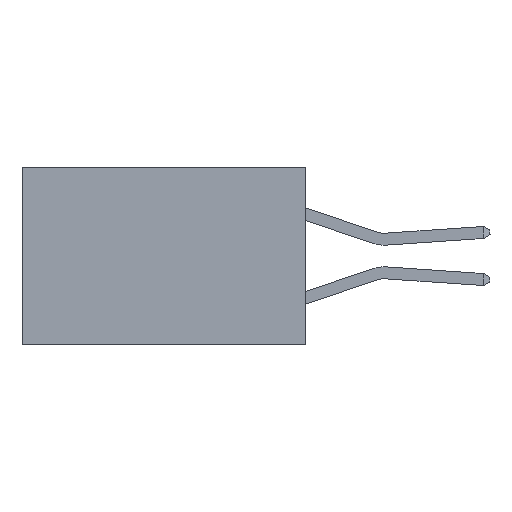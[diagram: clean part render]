
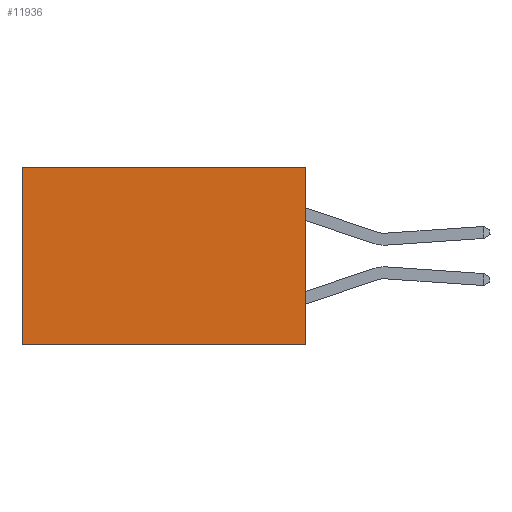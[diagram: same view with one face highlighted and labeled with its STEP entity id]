
A CAD part, left-side view. The second image highlights one B-rep face of the part: STEP entity #11936.
In plain terms, the highlighted planar face has unit normal (-1, 0, 0).
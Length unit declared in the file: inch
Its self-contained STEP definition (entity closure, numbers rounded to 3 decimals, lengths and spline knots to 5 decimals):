
#502 = ORIENTED_EDGE ( 'NONE', *, *, #6979, .T. ) ;
#2193 = AXIS2_PLACEMENT_3D ( 'NONE', #5976, #7230, #16061 ) ;
#3953 = ORIENTED_EDGE ( 'NONE', *, *, #11478, .F. ) ;
#5314 = LINE ( 'NONE', #7444, #8252 ) ;
#5525 = VERTEX_POINT ( 'NONE', #14274 ) ;
#5553 = ORIENTED_EDGE ( 'NONE', *, *, #6121, .T. ) ;
#5976 = CARTESIAN_POINT ( 'NONE',  ( 0.277, 0., -0.37 ) ) ;
#6121 = EDGE_CURVE ( 'NONE', #5525, #10886, #5314, .T. ) ;
#6979 = EDGE_CURVE ( 'NONE', #10886, #8081, #8620, .T. ) ;
#7230 = DIRECTION ( 'NONE',  ( 1., 0., 0. ) ) ;
#7444 = CARTESIAN_POINT ( 'NONE',  ( 0.277, 0., 0. ) ) ;
#7464 = EDGE_CURVE ( 'NONE', #5525, #8559, #8432, .T. ) ;
#7705 = ORIENTED_EDGE ( 'NONE', *, *, #7464, .F. ) ;
#8081 = VERTEX_POINT ( 'NONE', #8588 ) ;
#8252 = VECTOR ( 'NONE', #9541, 39.37008 ) ;
#8432 = LINE ( 'NONE', #10288, #15152 ) ;
#8559 = VERTEX_POINT ( 'NONE', #15080 ) ;
#8588 = CARTESIAN_POINT ( 'NONE',  ( 0.277, 0.59, -0.37 ) ) ;
#8620 = LINE ( 'NONE', #12965, #11882 ) ;
#9541 = DIRECTION ( 'NONE',  ( 0., 1., 0. ) ) ;
#9737 = PLANE ( 'NONE',  #2193 ) ;
#10176 = DIRECTION ( 'NONE',  ( 0., 0., -1. ) ) ;
#10288 = CARTESIAN_POINT ( 'NONE',  ( 0.277, 0., -0.37 ) ) ;
#10677 = LINE ( 'NONE', #14971, #16147 ) ;
#10886 = VERTEX_POINT ( 'NONE', #12755 ) ;
#11478 = EDGE_CURVE ( 'NONE', #8559, #8081, #10677, .T. ) ;
#11882 = VECTOR ( 'NONE', #12638, 39.37008 ) ;
#11936 = ADVANCED_FACE ( 'NONE', ( #15759 ), #9737, .F. ) ;
#12638 = DIRECTION ( 'NONE',  ( 0., 0., -1. ) ) ;
#12755 = CARTESIAN_POINT ( 'NONE',  ( 0.277, 0.59, 0. ) ) ;
#12965 = CARTESIAN_POINT ( 'NONE',  ( 0.277, 0.59, -0.37 ) ) ;
#13239 = EDGE_LOOP ( 'NONE', ( #502, #3953, #7705, #5553 ) ) ;
#14274 = CARTESIAN_POINT ( 'NONE',  ( 0.277, 0., 0. ) ) ;
#14971 = CARTESIAN_POINT ( 'NONE',  ( 0.277, 0., -0.37 ) ) ;
#15080 = CARTESIAN_POINT ( 'NONE',  ( 0.277, 0., -0.37 ) ) ;
#15152 = VECTOR ( 'NONE', #10176, 39.37008 ) ;
#15759 = FACE_OUTER_BOUND ( 'NONE', #13239, .T. ) ;
#16061 = DIRECTION ( 'NONE',  ( 0., 0., -1. ) ) ;
#16147 = VECTOR ( 'NONE', #16224, 39.37008 ) ;
#16224 = DIRECTION ( 'NONE',  ( 0., 1., 0. ) ) ;
